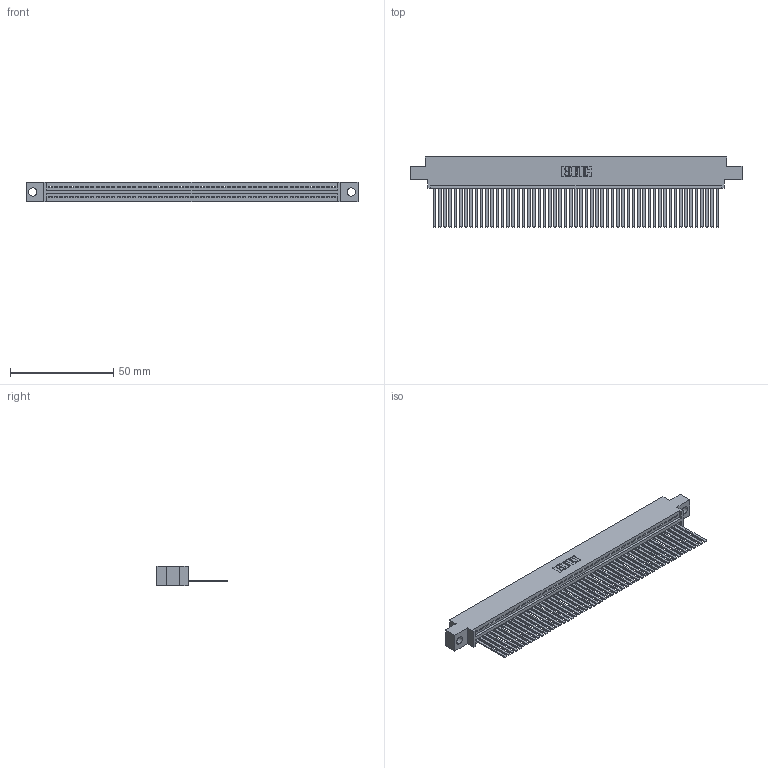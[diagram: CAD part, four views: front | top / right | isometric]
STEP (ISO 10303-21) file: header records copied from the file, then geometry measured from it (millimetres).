
FILE_DESCRIPTION (( 'STEP AP203' ), '1' );
FILE_NAME ('345-055-544-604.STEP', '2019-10-10T04:12:07', ( '' ), ( '' ), 'SwSTEP 2.0', 'SolidWorks 2016', '' );
FILE_SCHEMA (( 'CONFIG_CONTROL_DESIGN' ));
Length unit declared in the file: inch
Products named in the file (3): 345 Part_0.170 Offset - 0.156 Dia-TH; 345-055-544-604; 345-292-001_345-293-144
Assembly tree (56 placements, depth 2):
  345-055-544-604
    345 Part_0.170 Offset - 0.156 Dia-TH
    345-292-001_345-293-144  x55
Bounding box: 160.91 x 33.96 x 9.4 mm (x, y, z)
Volume: 15825.5 mm3; surface area: 23054.9 mm2
Topology: 56 solids, 56 shells, 2990 faces, 9043 edges, 5954 vertices
Faces by surface type: plane 2064, cylinder 926
Entity records: 39595 total; most frequent: CARTESIAN_POINT 6865, ORIENTED_EDGE 6854, DIRECTION 5973, EDGE_CURVE 3427, LINE 3079, VECTOR 3079, VERTEX_POINT 2282, AXIS2_PLACEMENT_3D 1447
